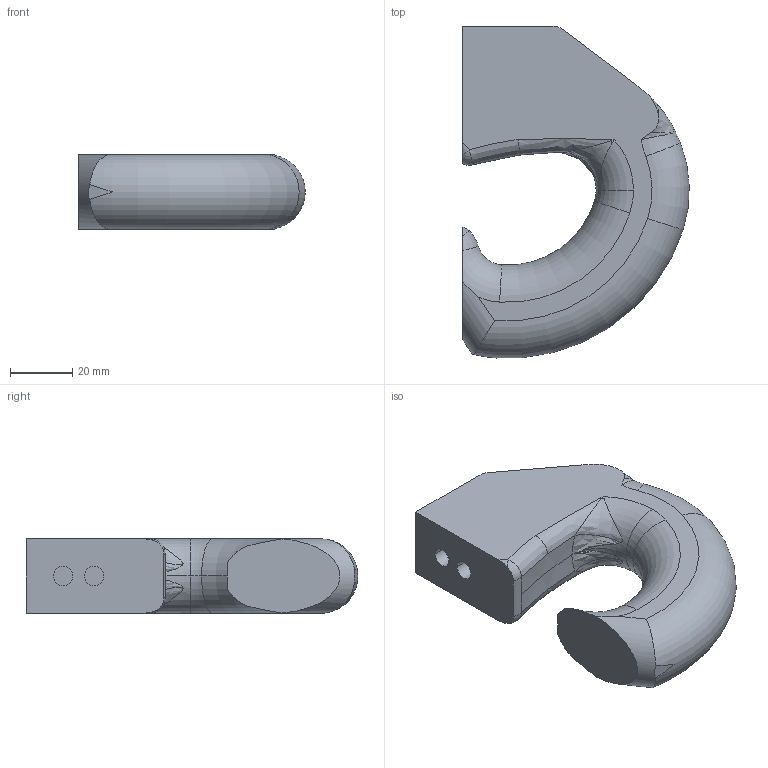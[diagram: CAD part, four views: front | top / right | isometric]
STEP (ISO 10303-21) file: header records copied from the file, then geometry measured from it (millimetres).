
FILE_DESCRIPTION (( 'STEP AP214' ), '1' );
FILE_NAME ('Receiver_Grip_1.step', '2014-05-14T06:10:14', ( 'WarFairy' ), ( '' ), 'SwSTEP 2.0', 'SolidWorks 2013', '' );
FILE_SCHEMA (( 'AUTOMOTIVE_DESIGN' ));
Length unit declared in the file: inch
Products named in the file (1): Receiver_Grip_1
Bounding box: 72.92 x 106.84 x 24 mm (x, y, z)
Volume: 108194.4 mm3; surface area: 17938.9 mm2
Topology: 1 solids, 1 shells, 60 faces, 154 edges, 92 vertices
Faces by surface type: bspline 22, cylinder 13, torus 12, plane 9, sphere 4
Entity records: 3631 total; most frequent: CARTESIAN_POINT 2317, ORIENTED_EDGE 296, DIRECTION 239, EDGE_CURVE 148, AXIS2_PLACEMENT_3D 108, VERTEX_POINT 92, CIRCLE 69, EDGE_LOOP 62
